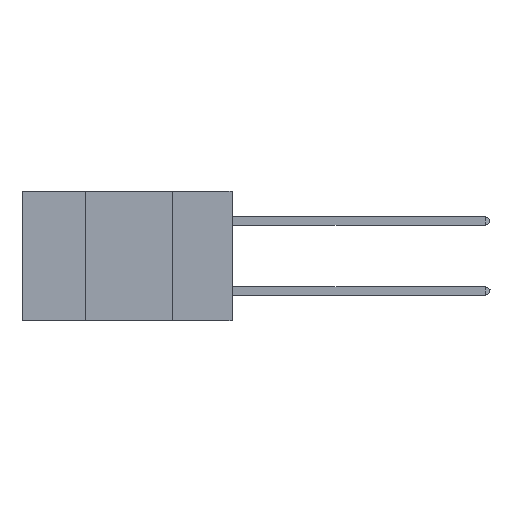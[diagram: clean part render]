
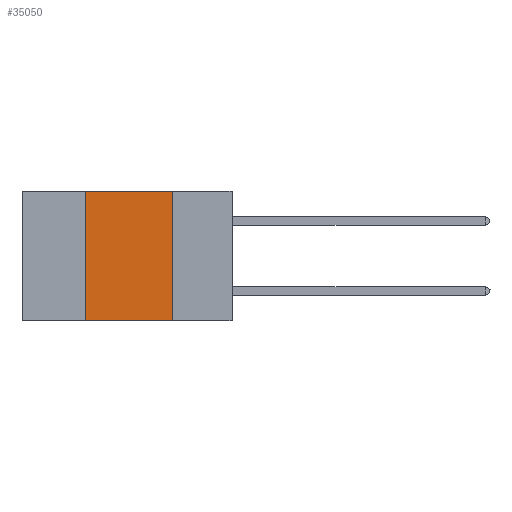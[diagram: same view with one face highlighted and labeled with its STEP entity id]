
A CAD part, left-side view. The second image highlights one B-rep face of the part: STEP entity #35050.
In plain terms, the highlighted planar face has unit normal (-1, 0, 0).
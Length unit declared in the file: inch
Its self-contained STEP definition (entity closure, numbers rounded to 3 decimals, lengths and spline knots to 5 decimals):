
#1575 = LINE ( 'NONE', #15627, #31237 ) ;
#3630 = EDGE_LOOP ( 'NONE', ( #4868, #12835, #13827, #35861 ) ) ;
#3684 = DIRECTION ( 'NONE',  ( 1., 0., 0. ) ) ;
#4059 = VERTEX_POINT ( 'NONE', #33014 ) ;
#4868 = ORIENTED_EDGE ( 'NONE', *, *, #9533, .F. ) ;
#6042 = DIRECTION ( 'NONE',  ( 0., -1., 0. ) ) ;
#6390 = FACE_OUTER_BOUND ( 'NONE', #3630, .T. ) ;
#7030 = VERTEX_POINT ( 'NONE', #36703 ) ;
#8144 = CARTESIAN_POINT ( 'NONE',  ( 0., 0.42, -0.37 ) ) ;
#9095 = AXIS2_PLACEMENT_3D ( 'NONE', #12918, #3684, #12345 ) ;
#9533 = EDGE_CURVE ( 'NONE', #4059, #7030, #1575, .T. ) ;
#11369 = DIRECTION ( 'NONE',  ( 0., 0., 1. ) ) ;
#11401 = VERTEX_POINT ( 'NONE', #33605 ) ;
#11504 = VECTOR ( 'NONE', #6042, 39.37008 ) ;
#12345 = DIRECTION ( 'NONE',  ( 0., 0., -1. ) ) ;
#12835 = ORIENTED_EDGE ( 'NONE', *, *, #25869, .F. ) ;
#12918 = CARTESIAN_POINT ( 'NONE',  ( 0., 0.6, 0. ) ) ;
#13121 = DIRECTION ( 'NONE',  ( 0., 0., -1. ) ) ;
#13645 = LINE ( 'NONE', #31489, #29032 ) ;
#13827 = ORIENTED_EDGE ( 'NONE', *, *, #28549, .F. ) ;
#15627 = CARTESIAN_POINT ( 'NONE',  ( 0., 0.17, 0. ) ) ;
#17479 = LINE ( 'NONE', #23592, #21347 ) ;
#17576 = LINE ( 'NONE', #35559, #11504 ) ;
#17982 = VERTEX_POINT ( 'NONE', #8144 ) ;
#21347 = VECTOR ( 'NONE', #29344, 39.37008 ) ;
#23592 = CARTESIAN_POINT ( 'NONE',  ( 0., 0.6, 0. ) ) ;
#24950 = EDGE_CURVE ( 'NONE', #17982, #7030, #17576, .T. ) ;
#25869 = EDGE_CURVE ( 'NONE', #11401, #4059, #17479, .T. ) ;
#28549 = EDGE_CURVE ( 'NONE', #17982, #11401, #13645, .T. ) ;
#29032 = VECTOR ( 'NONE', #11369, 39.37008 ) ;
#29344 = DIRECTION ( 'NONE',  ( 0., -1., 0. ) ) ;
#31237 = VECTOR ( 'NONE', #13121, 39.37008 ) ;
#31489 = CARTESIAN_POINT ( 'NONE',  ( 0., 0.42, 0. ) ) ;
#32855 = PLANE ( 'NONE',  #9095 ) ;
#33014 = CARTESIAN_POINT ( 'NONE',  ( 0., 0.17, 0. ) ) ;
#33605 = CARTESIAN_POINT ( 'NONE',  ( 0., 0.42, 0. ) ) ;
#35050 = ADVANCED_FACE ( 'NONE', ( #6390 ), #32855, .F. ) ;
#35559 = CARTESIAN_POINT ( 'NONE',  ( 0., 0.6, -0.37 ) ) ;
#35861 = ORIENTED_EDGE ( 'NONE', *, *, #24950, .T. ) ;
#36703 = CARTESIAN_POINT ( 'NONE',  ( 0., 0.17, -0.37 ) ) ;
